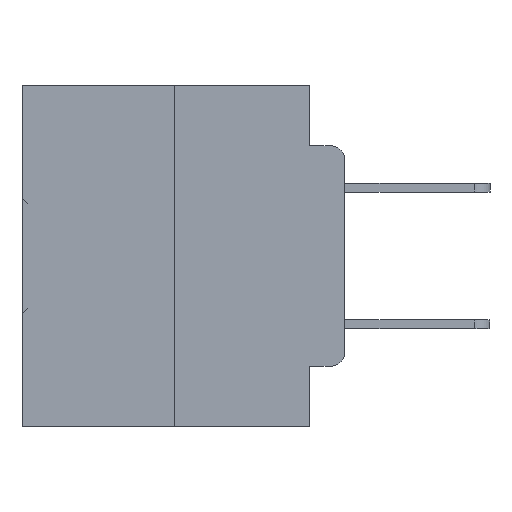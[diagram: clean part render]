
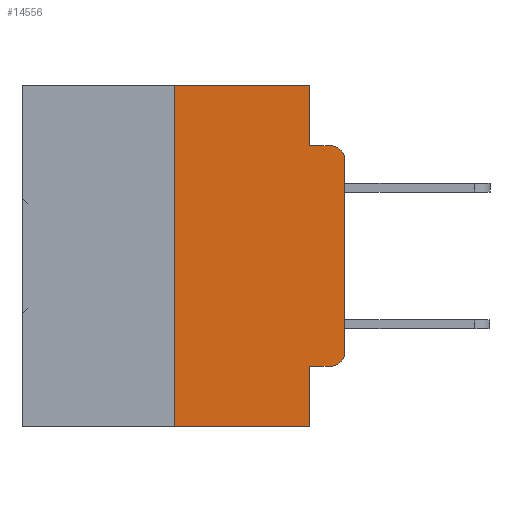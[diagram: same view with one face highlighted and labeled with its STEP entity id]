
A CAD part, left-side view. The second image highlights one B-rep face of the part: STEP entity #14556.
In plain terms, the highlighted planar face has unit normal (-1, 0, 0).
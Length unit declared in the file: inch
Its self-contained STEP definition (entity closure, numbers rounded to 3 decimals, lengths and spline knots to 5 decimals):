
#93 = AXIS2_PLACEMENT_3D ( 'NONE', #23265, #6742, #26038 ) ;
#307 = DIRECTION ( 'NONE',  ( 0., 0., -1. ) ) ;
#1180 = ORIENTED_EDGE ( 'NONE', *, *, #20446, .F. ) ;
#1631 = EDGE_CURVE ( 'NONE', #7939, #10404, #27459, .T. ) ;
#1718 = DIRECTION ( 'NONE',  ( 0., 0., -1. ) ) ;
#1843 = CARTESIAN_POINT ( 'NONE',  ( 0., 0.02, -0.0885 ) ) ;
#2120 = AXIS2_PLACEMENT_3D ( 'NONE', #13189, #11941, #307 ) ;
#2360 = EDGE_CURVE ( 'NONE', #6493, #4936, #27830, .T. ) ;
#3745 = EDGE_LOOP ( 'NONE', ( #34410, #6968, #1180, #10473, #26829, #5667, #35698, #9170, #10938, #5250 ) ) ;
#4095 = DIRECTION ( 'NONE',  ( 0., 0., -1. ) ) ;
#4115 = DIRECTION ( 'NONE',  ( 0., -1., 0. ) ) ;
#4256 = FACE_OUTER_BOUND ( 'NONE', #3745, .T. ) ;
#4415 = EDGE_CURVE ( 'NONE', #8002, #14842, #29237, .T. ) ;
#4615 = DIRECTION ( 'NONE',  ( 0., 0., -1. ) ) ;
#4887 = VECTOR ( 'NONE', #27127, 39.37008 ) ;
#4936 = VERTEX_POINT ( 'NONE', #33403 ) ;
#5070 = VERTEX_POINT ( 'NONE', #14953 ) ;
#5250 = ORIENTED_EDGE ( 'NONE', *, *, #2360, .T. ) ;
#5631 = VECTOR ( 'NONE', #6415, 39.37008 ) ;
#5657 = LINE ( 'NONE', #5731, #18584 ) ;
#5667 = ORIENTED_EDGE ( 'NONE', *, *, #1631, .F. ) ;
#5731 = CARTESIAN_POINT ( 'NONE',  ( 0., 0., 0. ) ) ;
#5845 = DIRECTION ( 'NONE',  ( 0., 0., 1. ) ) ;
#6236 = VECTOR ( 'NONE', #4115, 39.37008 ) ;
#6347 = LINE ( 'NONE', #18338, #20178 ) ;
#6415 = DIRECTION ( 'NONE',  ( 0., -1., 0. ) ) ;
#6493 = VERTEX_POINT ( 'NONE', #30138 ) ;
#6742 = DIRECTION ( 'NONE',  ( -1., 0., 0. ) ) ;
#6968 = ORIENTED_EDGE ( 'NONE', *, *, #18407, .T. ) ;
#7088 = EDGE_CURVE ( 'NONE', #7939, #5070, #21333, .T. ) ;
#7939 = VERTEX_POINT ( 'NONE', #29244 ) ;
#8002 = VERTEX_POINT ( 'NONE', #34870 ) ;
#8551 = EDGE_CURVE ( 'NONE', #10404, #8002, #24718, .T. ) ;
#9170 = ORIENTED_EDGE ( 'NONE', *, *, #24667, .F. ) ;
#9691 = CARTESIAN_POINT ( 'NONE',  ( 0., 0., -0.1085 ) ) ;
#10104 = CARTESIAN_POINT ( 'NONE',  ( 0., 0.473, 0. ) ) ;
#10119 = VERTEX_POINT ( 'NONE', #1843 ) ;
#10404 = VERTEX_POINT ( 'NONE', #11927 ) ;
#10473 = ORIENTED_EDGE ( 'NONE', *, *, #4415, .F. ) ;
#10938 = ORIENTED_EDGE ( 'NONE', *, *, #17228, .T. ) ;
#11927 = CARTESIAN_POINT ( 'NONE',  ( 0., 0.25, 0. ) ) ;
#11941 = DIRECTION ( 'NONE',  ( -1., 0., 0. ) ) ;
#11999 = CARTESIAN_POINT ( 'NONE',  ( 0., 0.051, -0.4115 ) ) ;
#12641 = DIRECTION ( 'NONE',  ( 0., -1., 0. ) ) ;
#12911 = DIRECTION ( 'NONE',  ( 0., 0., 1. ) ) ;
#13031 = LINE ( 'NONE', #28330, #5631 ) ;
#13067 = VERTEX_POINT ( 'NONE', #11999 ) ;
#13189 = CARTESIAN_POINT ( 'NONE',  ( 0., 0.02, -0.3915 ) ) ;
#13625 = LINE ( 'NONE', #31567, #6236 ) ;
#13688 = AXIS2_PLACEMENT_3D ( 'NONE', #10104, #18349, #1718 ) ;
#14556 = ADVANCED_FACE ( 'NONE', ( #4256 ), #34729, .F. ) ;
#14842 = VERTEX_POINT ( 'NONE', #22465 ) ;
#14953 = CARTESIAN_POINT ( 'NONE',  ( 0., 0.051, -0.5 ) ) ;
#15352 = CARTESIAN_POINT ( 'NONE',  ( 0., 0.473, 0. ) ) ;
#17228 = EDGE_CURVE ( 'NONE', #13067, #6493, #13625, .T. ) ;
#17338 = VECTOR ( 'NONE', #12641, 39.37008 ) ;
#18015 = VECTOR ( 'NONE', #4095, 39.37008 ) ;
#18338 = CARTESIAN_POINT ( 'NONE',  ( 0., 0.051, 0. ) ) ;
#18349 = DIRECTION ( 'NONE',  ( 1., 0., 0. ) ) ;
#18407 = EDGE_CURVE ( 'NONE', #32154, #10119, #18646, .T. ) ;
#18584 = VECTOR ( 'NONE', #5845, 39.37008 ) ;
#18646 = CIRCLE ( 'NONE', #93, 0.02 ) ;
#20178 = VECTOR ( 'NONE', #4615, 39.37008 ) ;
#20446 = EDGE_CURVE ( 'NONE', #14842, #10119, #13031, .T. ) ;
#21333 = LINE ( 'NONE', #35138, #4887 ) ;
#22465 = CARTESIAN_POINT ( 'NONE',  ( 0., 0.051, -0.0885 ) ) ;
#23265 = CARTESIAN_POINT ( 'NONE',  ( 0., 0.02, -0.1085 ) ) ;
#23426 = CARTESIAN_POINT ( 'NONE',  ( 0., 0.051, 0. ) ) ;
#24667 = EDGE_CURVE ( 'NONE', #13067, #5070, #6347, .T. ) ;
#24718 = LINE ( 'NONE', #15352, #17338 ) ;
#26038 = DIRECTION ( 'NONE',  ( 0., 0., -1. ) ) ;
#26599 = CARTESIAN_POINT ( 'NONE',  ( 0., 0.25, 0. ) ) ;
#26829 = ORIENTED_EDGE ( 'NONE', *, *, #8551, .F. ) ;
#27127 = DIRECTION ( 'NONE',  ( 0., -1., 0. ) ) ;
#27459 = LINE ( 'NONE', #26599, #35481 ) ;
#27830 = CIRCLE ( 'NONE', #2120, 0.02 ) ;
#28011 = EDGE_CURVE ( 'NONE', #4936, #32154, #5657, .T. ) ;
#28330 = CARTESIAN_POINT ( 'NONE',  ( 0., 0.051, -0.0885 ) ) ;
#29237 = LINE ( 'NONE', #23426, #18015 ) ;
#29244 = CARTESIAN_POINT ( 'NONE',  ( 0., 0.25, -0.5 ) ) ;
#30138 = CARTESIAN_POINT ( 'NONE',  ( 0., 0.02, -0.4115 ) ) ;
#31567 = CARTESIAN_POINT ( 'NONE',  ( 0., 0.051, -0.4115 ) ) ;
#32154 = VERTEX_POINT ( 'NONE', #9691 ) ;
#33403 = CARTESIAN_POINT ( 'NONE',  ( 0., 0., -0.3915 ) ) ;
#34410 = ORIENTED_EDGE ( 'NONE', *, *, #28011, .T. ) ;
#34729 = PLANE ( 'NONE',  #13688 ) ;
#34870 = CARTESIAN_POINT ( 'NONE',  ( 0., 0.051, 0. ) ) ;
#35138 = CARTESIAN_POINT ( 'NONE',  ( 0., 0.473, -0.5 ) ) ;
#35481 = VECTOR ( 'NONE', #12911, 39.37008 ) ;
#35698 = ORIENTED_EDGE ( 'NONE', *, *, #7088, .T. ) ;
